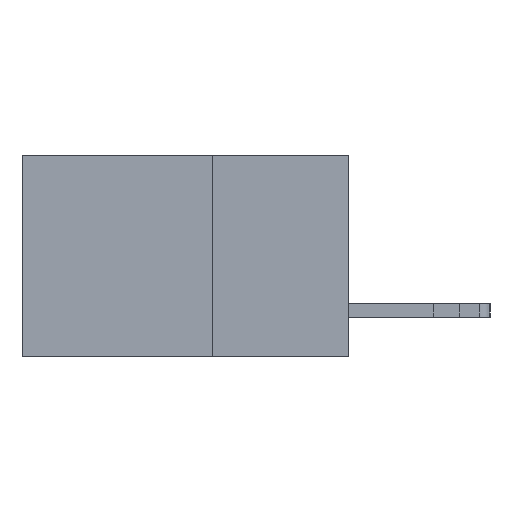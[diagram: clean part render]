
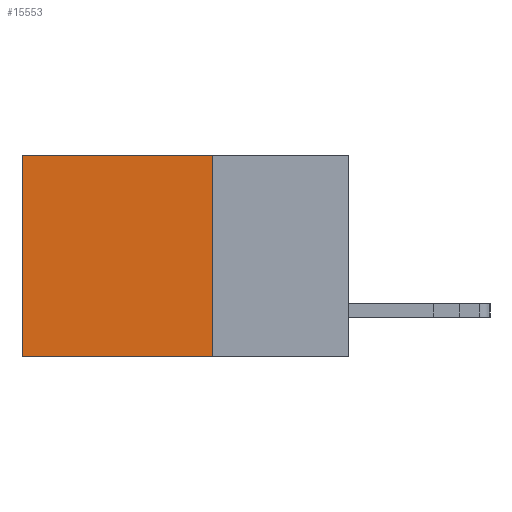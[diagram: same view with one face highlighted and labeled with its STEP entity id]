
A CAD part, left-side view. The second image highlights one B-rep face of the part: STEP entity #15553.
In plain terms, the highlighted planar face has unit normal (-1, 0, 0).
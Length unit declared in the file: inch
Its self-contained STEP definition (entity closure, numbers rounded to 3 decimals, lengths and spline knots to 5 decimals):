
#541 = CARTESIAN_POINT ( 'NONE',  ( 0.298, 0.25, 0. ) ) ;
#988 = CARTESIAN_POINT ( 'NONE',  ( 0.298, 0.25, 0. ) ) ;
#1134 = VERTEX_POINT ( 'NONE', #11232 ) ;
#1338 = VECTOR ( 'NONE', #7491, 39.37008 ) ;
#2308 = EDGE_CURVE ( 'NONE', #18545, #10667, #10768, .T. ) ;
#2823 = LINE ( 'NONE', #541, #21230 ) ;
#3041 = CARTESIAN_POINT ( 'NONE',  ( 0.298, 0.6, -0.37 ) ) ;
#3719 = CARTESIAN_POINT ( 'NONE',  ( 0.298, 0.25, -0.37 ) ) ;
#3810 = EDGE_CURVE ( 'NONE', #1134, #19921, #2823, .T. ) ;
#3906 = PLANE ( 'NONE',  #18474 ) ;
#4999 = ORIENTED_EDGE ( 'NONE', *, *, #3810, .F. ) ;
#6669 = EDGE_CURVE ( 'NONE', #19921, #10667, #16106, .T. ) ;
#7491 = DIRECTION ( 'NONE',  ( 0., 1., 0. ) ) ;
#7677 = CARTESIAN_POINT ( 'NONE',  ( 0.298, 0.25, 0. ) ) ;
#8092 = EDGE_LOOP ( 'NONE', ( #17466, #8157, #4999, #10525 ) ) ;
#8157 = ORIENTED_EDGE ( 'NONE', *, *, #6669, .F. ) ;
#9503 = DIRECTION ( 'NONE',  ( 0., 0., -1. ) ) ;
#10525 = ORIENTED_EDGE ( 'NONE', *, *, #19801, .T. ) ;
#10667 = VERTEX_POINT ( 'NONE', #3041 ) ;
#10768 = LINE ( 'NONE', #19568, #19882 ) ;
#11232 = CARTESIAN_POINT ( 'NONE',  ( 0.298, 0.25, 0. ) ) ;
#11708 = FACE_OUTER_BOUND ( 'NONE', #8092, .T. ) ;
#12135 = DIRECTION ( 'NONE',  ( 0., 1., 0. ) ) ;
#14313 = VECTOR ( 'NONE', #12135, 39.37008 ) ;
#14403 = CARTESIAN_POINT ( 'NONE',  ( 0.298, 0.25, -0.37 ) ) ;
#15553 = ADVANCED_FACE ( 'NONE', ( #11708 ), #3906, .F. ) ;
#16106 = LINE ( 'NONE', #3719, #1338 ) ;
#17112 = DIRECTION ( 'NONE',  ( 0., 0., -1. ) ) ;
#17466 = ORIENTED_EDGE ( 'NONE', *, *, #2308, .T. ) ;
#18474 = AXIS2_PLACEMENT_3D ( 'NONE', #7677, #20448, #9503 ) ;
#18545 = VERTEX_POINT ( 'NONE', #19557 ) ;
#19087 = LINE ( 'NONE', #988, #14313 ) ;
#19557 = CARTESIAN_POINT ( 'NONE',  ( 0.298, 0.6, 0. ) ) ;
#19568 = CARTESIAN_POINT ( 'NONE',  ( 0.298, 0.6, 0. ) ) ;
#19593 = DIRECTION ( 'NONE',  ( 0., 0., -1. ) ) ;
#19801 = EDGE_CURVE ( 'NONE', #1134, #18545, #19087, .T. ) ;
#19882 = VECTOR ( 'NONE', #19593, 39.37008 ) ;
#19921 = VERTEX_POINT ( 'NONE', #14403 ) ;
#20448 = DIRECTION ( 'NONE',  ( 1., 0., 0. ) ) ;
#21230 = VECTOR ( 'NONE', #17112, 39.37008 ) ;
